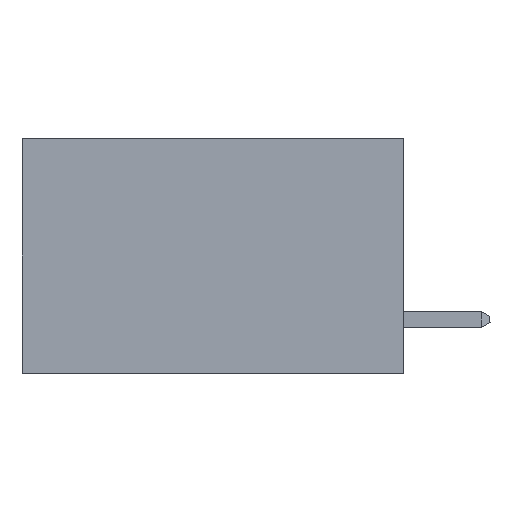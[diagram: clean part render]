
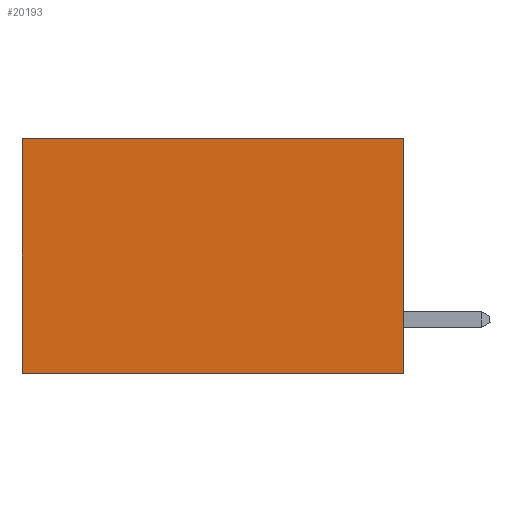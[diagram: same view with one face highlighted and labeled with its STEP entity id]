
A CAD part, left-side view. The second image highlights one B-rep face of the part: STEP entity #20193.
In plain terms, the highlighted planar face has unit normal (-1, 0, 0).
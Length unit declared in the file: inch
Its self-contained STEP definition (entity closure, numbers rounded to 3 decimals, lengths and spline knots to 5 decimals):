
#499 = CARTESIAN_POINT ( 'NONE',  ( 0.2875, 0., -0.37 ) ) ;
#617 = CARTESIAN_POINT ( 'NONE',  ( 0.2875, 0., 0. ) ) ;
#1249 = DIRECTION ( 'NONE',  ( 0., 0., -1. ) ) ;
#1894 = CARTESIAN_POINT ( 'NONE',  ( 0.2875, 0.6, -0.37 ) ) ;
#1954 = ORIENTED_EDGE ( 'NONE', *, *, #2197, .T. ) ;
#2197 = EDGE_CURVE ( 'NONE', #9843, #19647, #8814, .T. ) ;
#2201 = ORIENTED_EDGE ( 'NONE', *, *, #19407, .F. ) ;
#2354 = DIRECTION ( 'NONE',  ( 0., 1., 0. ) ) ;
#2593 = FACE_OUTER_BOUND ( 'NONE', #15673, .T. ) ;
#3013 = VERTEX_POINT ( 'NONE', #9475 ) ;
#4289 = LINE ( 'NONE', #11885, #13600 ) ;
#4758 = VECTOR ( 'NONE', #17823, 39.37008 ) ;
#4861 = CARTESIAN_POINT ( 'NONE',  ( 0.2875, 0.6, 0. ) ) ;
#7107 = VERTEX_POINT ( 'NONE', #617 ) ;
#7219 = PLANE ( 'NONE',  #16273 ) ;
#7480 = CARTESIAN_POINT ( 'NONE',  ( 0.2875, 0., 0. ) ) ;
#8273 = VECTOR ( 'NONE', #15934, 39.37008 ) ;
#8814 = LINE ( 'NONE', #21410, #8273 ) ;
#8907 = LINE ( 'NONE', #7480, #4758 ) ;
#9475 = CARTESIAN_POINT ( 'NONE',  ( 0.2875, 0., -0.37 ) ) ;
#9843 = VERTEX_POINT ( 'NONE', #4861 ) ;
#10722 = DIRECTION ( 'NONE',  ( 0., 0., -1. ) ) ;
#11885 = CARTESIAN_POINT ( 'NONE',  ( 0.2875, 0., 0. ) ) ;
#13117 = EDGE_CURVE ( 'NONE', #3013, #19647, #18834, .T. ) ;
#13600 = VECTOR ( 'NONE', #1249, 39.37008 ) ;
#15673 = EDGE_LOOP ( 'NONE', ( #1954, #20057, #2201, #16425 ) ) ;
#15934 = DIRECTION ( 'NONE',  ( 0., 0., -1. ) ) ;
#16273 = AXIS2_PLACEMENT_3D ( 'NONE', #19299, #21054, #10722 ) ;
#16425 = ORIENTED_EDGE ( 'NONE', *, *, #21799, .T. ) ;
#17755 = VECTOR ( 'NONE', #2354, 39.37008 ) ;
#17823 = DIRECTION ( 'NONE',  ( 0., 1., 0. ) ) ;
#18834 = LINE ( 'NONE', #499, #17755 ) ;
#19299 = CARTESIAN_POINT ( 'NONE',  ( 0.2875, 0., 0. ) ) ;
#19407 = EDGE_CURVE ( 'NONE', #7107, #3013, #4289, .T. ) ;
#19647 = VERTEX_POINT ( 'NONE', #1894 ) ;
#20057 = ORIENTED_EDGE ( 'NONE', *, *, #13117, .F. ) ;
#20193 = ADVANCED_FACE ( 'NONE', ( #2593 ), #7219, .F. ) ;
#21054 = DIRECTION ( 'NONE',  ( 1., 0., 0. ) ) ;
#21410 = CARTESIAN_POINT ( 'NONE',  ( 0.2875, 0.6, 0. ) ) ;
#21799 = EDGE_CURVE ( 'NONE', #7107, #9843, #8907, .T. ) ;
